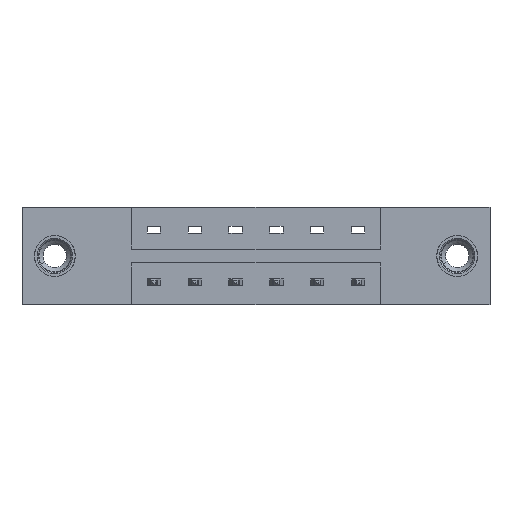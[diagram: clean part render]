
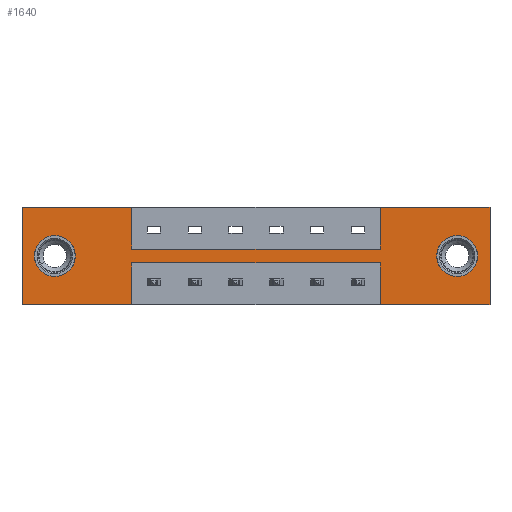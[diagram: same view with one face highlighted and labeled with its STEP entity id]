
A CAD part, front view. The second image highlights one B-rep face of the part: STEP entity #1640.
In plain terms, the highlighted planar face has unit normal (0, -1, 0).
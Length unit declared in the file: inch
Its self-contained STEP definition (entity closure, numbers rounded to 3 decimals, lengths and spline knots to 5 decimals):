
#6 = EDGE_CURVE ( 'NONE', #4030, #8530, #2349, .T. ) ;
#62 = EDGE_CURVE ( 'NONE', #2721, #8078, #3317, .T. ) ;
#117 = ORIENTED_EDGE ( 'NONE', *, *, #5791, .F. ) ;
#159 = LINE ( 'NONE', #6054, #3286 ) ;
#187 = ORIENTED_EDGE ( 'NONE', *, *, #4499, .F. ) ;
#252 = CARTESIAN_POINT ( 'NONE',  ( 1.3665, 0., 0. ) ) ;
#274 = DIRECTION ( 'NONE',  ( 0., 0., 1. ) ) ;
#360 = DIRECTION ( 'NONE',  ( 0., 0., -1. ) ) ;
#376 = AXIS2_PLACEMENT_3D ( 'NONE', #6115, #3900, #9057 ) ;
#560 = ORIENTED_EDGE ( 'NONE', *, *, #6591, .T. ) ;
#620 = CARTESIAN_POINT ( 'NONE',  ( 0.4175, 0., -0.2115 ) ) ;
#670 = CARTESIAN_POINT ( 'NONE',  ( 1.659, 0., -0.107 ) ) ;
#705 = ORIENTED_EDGE ( 'NONE', *, *, #6, .T. ) ;
#716 = EDGE_CURVE ( 'NONE', #8143, #2086, #4604, .T. ) ;
#721 = ORIENTED_EDGE ( 'NONE', *, *, #9259, .F. ) ;
#736 = CARTESIAN_POINT ( 'NONE',  ( 0.125, 0., -0.263 ) ) ;
#758 = VERTEX_POINT ( 'NONE', #9035 ) ;
#834 = DIRECTION ( 'NONE',  ( 0., 0., -1. ) ) ;
#849 = VERTEX_POINT ( 'NONE', #4887 ) ;
#937 = CARTESIAN_POINT ( 'NONE',  ( 0., 0., -0.37 ) ) ;
#1006 = CARTESIAN_POINT ( 'NONE',  ( 0., 0., 0. ) ) ;
#1011 = VECTOR ( 'NONE', #2749, 39.37008 ) ;
#1056 = CARTESIAN_POINT ( 'NONE',  ( 1.3665, 0., -0.1585 ) ) ;
#1062 = CARTESIAN_POINT ( 'NONE',  ( 1.3665, 0., -0.2115 ) ) ;
#1145 = CIRCLE ( 'NONE', #7138, 0.078 ) ;
#1256 = LINE ( 'NONE', #8197, #6964 ) ;
#1506 = CARTESIAN_POINT ( 'NONE',  ( 0.4175, 0., 0. ) ) ;
#1511 = ORIENTED_EDGE ( 'NONE', *, *, #3714, .F. ) ;
#1518 = VECTOR ( 'NONE', #3972, 39.37008 ) ;
#1522 = ORIENTED_EDGE ( 'NONE', *, *, #6278, .T. ) ;
#1526 = VERTEX_POINT ( 'NONE', #5097 ) ;
#1640 = ADVANCED_FACE ( 'NONE', ( #3851, #6779, #4674 ), #2326, .T. ) ;
#1706 = ORIENTED_EDGE ( 'NONE', *, *, #62, .F. ) ;
#1733 = VECTOR ( 'NONE', #7023, 39.37008 ) ;
#1745 = CARTESIAN_POINT ( 'NONE',  ( 0., 0., -0.37 ) ) ;
#1924 = VERTEX_POINT ( 'NONE', #5904 ) ;
#2003 = CARTESIAN_POINT ( 'NONE',  ( 0.125, 0., -0.107 ) ) ;
#2017 = CARTESIAN_POINT ( 'NONE',  ( 1.659, 0., -0.263 ) ) ;
#2086 = VERTEX_POINT ( 'NONE', #3200 ) ;
#2152 = DIRECTION ( 'NONE',  ( 0., 0., -1. ) ) ;
#2326 = PLANE ( 'NONE',  #5335 ) ;
#2349 = CIRCLE ( 'NONE', #2966, 0.078 ) ;
#2398 = DIRECTION ( 'NONE',  ( 0., 1., 0. ) ) ;
#2408 = ORIENTED_EDGE ( 'NONE', *, *, #5568, .F. ) ;
#2556 = EDGE_CURVE ( 'NONE', #5980, #2721, #7609, .T. ) ;
#2587 = CARTESIAN_POINT ( 'NONE',  ( 1.784, 0., 0. ) ) ;
#2721 = VERTEX_POINT ( 'NONE', #5847 ) ;
#2749 = DIRECTION ( 'NONE',  ( -1., 0., 0. ) ) ;
#2797 = VERTEX_POINT ( 'NONE', #670 ) ;
#2846 = CARTESIAN_POINT ( 'NONE',  ( 1.784, 0., -0.37 ) ) ;
#2966 = AXIS2_PLACEMENT_3D ( 'NONE', #9018, #2398, #8297 ) ;
#3045 = EDGE_LOOP ( 'NONE', ( #560, #705 ) ) ;
#3107 = DIRECTION ( 'NONE',  ( -1., 0., 0. ) ) ;
#3165 = CARTESIAN_POINT ( 'NONE',  ( 0., 0., -0.37 ) ) ;
#3171 = ORIENTED_EDGE ( 'NONE', *, *, #716, .F. ) ;
#3200 = CARTESIAN_POINT ( 'NONE',  ( 1.3665, 0., -0.2115 ) ) ;
#3286 = VECTOR ( 'NONE', #8997, 39.37008 ) ;
#3317 = LINE ( 'NONE', #2587, #1733 ) ;
#3319 = VECTOR ( 'NONE', #7193, 39.37008 ) ;
#3427 = ORIENTED_EDGE ( 'NONE', *, *, #9105, .T. ) ;
#3541 = LINE ( 'NONE', #4283, #3319 ) ;
#3714 = EDGE_CURVE ( 'NONE', #6513, #5980, #9101, .T. ) ;
#3784 = EDGE_CURVE ( 'NONE', #5832, #1924, #8234, .T. ) ;
#3851 = FACE_BOUND ( 'NONE', #6628, .T. ) ;
#3900 = DIRECTION ( 'NONE',  ( 0., 1., 0. ) ) ;
#3972 = DIRECTION ( 'NONE',  ( 1., 0., 0. ) ) ;
#4025 = DIRECTION ( 'NONE',  ( 0., 0., 1. ) ) ;
#4030 = VERTEX_POINT ( 'NONE', #736 ) ;
#4080 = DIRECTION ( 'NONE',  ( 0., 1., 0. ) ) ;
#4118 = VERTEX_POINT ( 'NONE', #1506 ) ;
#4283 = CARTESIAN_POINT ( 'NONE',  ( 0.4175, 0., -0.2115 ) ) ;
#4363 = DIRECTION ( 'NONE',  ( 1., 0., 0. ) ) ;
#4499 = EDGE_CURVE ( 'NONE', #1924, #1526, #1256, .T. ) ;
#4552 = VERTEX_POINT ( 'NONE', #2017 ) ;
#4575 = CIRCLE ( 'NONE', #7470, 0.078 ) ;
#4604 = LINE ( 'NONE', #1062, #8860 ) ;
#4619 = LINE ( 'NONE', #1745, #8680 ) ;
#4634 = ORIENTED_EDGE ( 'NONE', *, *, #3784, .F. ) ;
#4668 = ORIENTED_EDGE ( 'NONE', *, *, #7315, .F. ) ;
#4674 = FACE_OUTER_BOUND ( 'NONE', #5944, .T. ) ;
#4761 = DIRECTION ( 'NONE',  ( 0., 0., -1. ) ) ;
#4887 = CARTESIAN_POINT ( 'NONE',  ( 0.4175, 0., -0.2115 ) ) ;
#5034 = CARTESIAN_POINT ( 'NONE',  ( 1.3665, 0., -0.37 ) ) ;
#5097 = CARTESIAN_POINT ( 'NONE',  ( 0., 0., 0. ) ) ;
#5325 = VECTOR ( 'NONE', #834, 39.37008 ) ;
#5333 = DIRECTION ( 'NONE',  ( -1., 0., 0. ) ) ;
#5335 = AXIS2_PLACEMENT_3D ( 'NONE', #937, #8288, #360 ) ;
#5562 = CARTESIAN_POINT ( 'NONE',  ( 1.659, 0., -0.185 ) ) ;
#5568 = EDGE_CURVE ( 'NONE', #758, #6513, #159, .T. ) ;
#5574 = EDGE_CURVE ( 'NONE', #8078, #8143, #4619, .T. ) ;
#5701 = CARTESIAN_POINT ( 'NONE',  ( 0.4175, 0., -0.37 ) ) ;
#5791 = EDGE_CURVE ( 'NONE', #1526, #4118, #6508, .T. ) ;
#5832 = VERTEX_POINT ( 'NONE', #5701 ) ;
#5846 = LINE ( 'NONE', #620, #1011 ) ;
#5847 = CARTESIAN_POINT ( 'NONE',  ( 1.784, 0., 0. ) ) ;
#5904 = CARTESIAN_POINT ( 'NONE',  ( 0., 0., -0.37 ) ) ;
#5944 = EDGE_LOOP ( 'NONE', ( #3171, #8930, #1706, #9307, #1511, #2408, #4668, #117, #187, #4634, #6045, #721 ) ) ;
#5980 = VERTEX_POINT ( 'NONE', #252 ) ;
#6045 = ORIENTED_EDGE ( 'NONE', *, *, #7542, .F. ) ;
#6054 = CARTESIAN_POINT ( 'NONE',  ( 0.4175, 0., -0.1585 ) ) ;
#6115 = CARTESIAN_POINT ( 'NONE',  ( 0.125, 0., -0.185 ) ) ;
#6278 = EDGE_CURVE ( 'NONE', #2797, #4552, #1145, .T. ) ;
#6508 = LINE ( 'NONE', #8063, #9001 ) ;
#6513 = VERTEX_POINT ( 'NONE', #1056 ) ;
#6557 = CARTESIAN_POINT ( 'NONE',  ( 1.659, 0., -0.185 ) ) ;
#6591 = EDGE_CURVE ( 'NONE', #8530, #4030, #8699, .T. ) ;
#6628 = EDGE_LOOP ( 'NONE', ( #1522, #3427 ) ) ;
#6779 = FACE_BOUND ( 'NONE', #3045, .T. ) ;
#6964 = VECTOR ( 'NONE', #9372, 39.37008 ) ;
#6990 = VECTOR ( 'NONE', #274, 39.37008 ) ;
#6999 = VECTOR ( 'NONE', #3107, 39.37008 ) ;
#7023 = DIRECTION ( 'NONE',  ( 0., 0., -1. ) ) ;
#7138 = AXIS2_PLACEMENT_3D ( 'NONE', #6557, #8778, #2152 ) ;
#7193 = DIRECTION ( 'NONE',  ( 0., 0., -1. ) ) ;
#7315 = EDGE_CURVE ( 'NONE', #4118, #758, #7389, .T. ) ;
#7389 = LINE ( 'NONE', #8178, #5325 ) ;
#7470 = AXIS2_PLACEMENT_3D ( 'NONE', #5562, #4080, #4761 ) ;
#7542 = EDGE_CURVE ( 'NONE', #849, #5832, #3541, .T. ) ;
#7594 = CARTESIAN_POINT ( 'NONE',  ( 1.3665, 0., -0.1585 ) ) ;
#7609 = LINE ( 'NONE', #1006, #1518 ) ;
#8063 = CARTESIAN_POINT ( 'NONE',  ( 0., 0., 0. ) ) ;
#8078 = VERTEX_POINT ( 'NONE', #2846 ) ;
#8143 = VERTEX_POINT ( 'NONE', #5034 ) ;
#8178 = CARTESIAN_POINT ( 'NONE',  ( 0.4175, 0., -0.1585 ) ) ;
#8197 = CARTESIAN_POINT ( 'NONE',  ( 0., 0., 0. ) ) ;
#8234 = LINE ( 'NONE', #3165, #6999 ) ;
#8288 = DIRECTION ( 'NONE',  ( 0., -1., 0. ) ) ;
#8297 = DIRECTION ( 'NONE',  ( 0., 0., 1. ) ) ;
#8530 = VERTEX_POINT ( 'NONE', #2003 ) ;
#8680 = VECTOR ( 'NONE', #5333, 39.37008 ) ;
#8699 = CIRCLE ( 'NONE', #376, 0.078 ) ;
#8778 = DIRECTION ( 'NONE',  ( 0., 1., 0. ) ) ;
#8860 = VECTOR ( 'NONE', #4025, 39.37008 ) ;
#8930 = ORIENTED_EDGE ( 'NONE', *, *, #5574, .F. ) ;
#8997 = DIRECTION ( 'NONE',  ( 1., 0., 0. ) ) ;
#9001 = VECTOR ( 'NONE', #4363, 39.37008 ) ;
#9018 = CARTESIAN_POINT ( 'NONE',  ( 0.125, 0., -0.185 ) ) ;
#9035 = CARTESIAN_POINT ( 'NONE',  ( 0.4175, 0., -0.1585 ) ) ;
#9057 = DIRECTION ( 'NONE',  ( 0., 0., 1. ) ) ;
#9101 = LINE ( 'NONE', #7594, #6990 ) ;
#9105 = EDGE_CURVE ( 'NONE', #4552, #2797, #4575, .T. ) ;
#9259 = EDGE_CURVE ( 'NONE', #2086, #849, #5846, .T. ) ;
#9307 = ORIENTED_EDGE ( 'NONE', *, *, #2556, .F. ) ;
#9372 = DIRECTION ( 'NONE',  ( 0., 0., 1. ) ) ;
